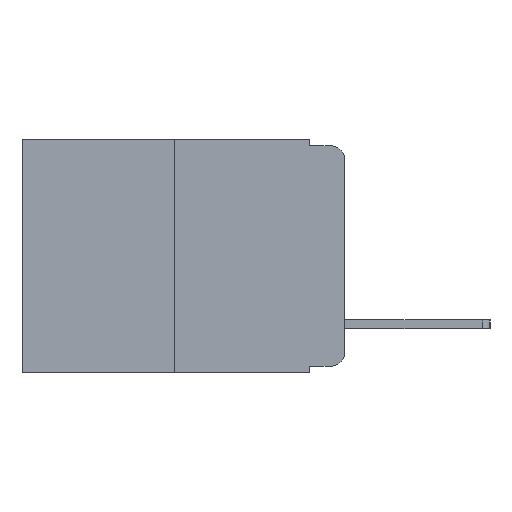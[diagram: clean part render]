
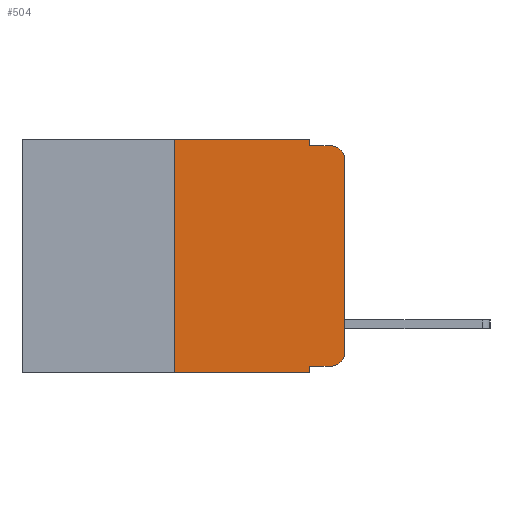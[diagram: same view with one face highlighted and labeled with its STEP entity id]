
A CAD part, left-side view. The second image highlights one B-rep face of the part: STEP entity #504.
In plain terms, the highlighted planar face has unit normal (-1, 0, 0).
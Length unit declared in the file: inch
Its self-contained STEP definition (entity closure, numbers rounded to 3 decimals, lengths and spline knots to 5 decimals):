
#94 = VERTEX_POINT ( 'NONE', #10260 ) ;
#504 = ADVANCED_FACE ( 'NONE', ( #7263 ), #11736, .F. ) ;
#627 = CARTESIAN_POINT ( 'NONE',  ( 0., 0.02, -0.01 ) ) ;
#659 = DIRECTION ( 'NONE',  ( 0., 0., 1. ) ) ;
#711 = CARTESIAN_POINT ( 'NONE',  ( 0., 0.051, 0. ) ) ;
#779 = VERTEX_POINT ( 'NONE', #1316 ) ;
#850 = DIRECTION ( 'NONE',  ( -1., 0., 0. ) ) ;
#1192 = EDGE_CURVE ( 'NONE', #10123, #94, #7740, .T. ) ;
#1227 = CIRCLE ( 'NONE', #11125, 0.02 ) ;
#1251 = VECTOR ( 'NONE', #8469, 39.37008 ) ;
#1261 = CARTESIAN_POINT ( 'NONE',  ( 0., 0., -0.03 ) ) ;
#1316 = CARTESIAN_POINT ( 'NONE',  ( 0., 0.051, -0.343 ) ) ;
#1371 = ORIENTED_EDGE ( 'NONE', *, *, #4126, .F. ) ;
#1494 = DIRECTION ( 'NONE',  ( 0., -1., 0. ) ) ;
#1604 = DIRECTION ( 'NONE',  ( -1., 0., 0. ) ) ;
#1645 = EDGE_LOOP ( 'NONE', ( #10729, #10468, #8356, #1371, #3718, #10208, #5669, #6054, #7855, #7959 ) ) ;
#1779 = VERTEX_POINT ( 'NONE', #7232 ) ;
#2030 = LINE ( 'NONE', #711, #6617 ) ;
#2799 = DIRECTION ( 'NONE',  ( 0., 0., -1. ) ) ;
#2885 = DIRECTION ( 'NONE',  ( 0., 0., -1. ) ) ;
#3276 = VECTOR ( 'NONE', #7156, 39.37008 ) ;
#3371 = EDGE_CURVE ( 'NONE', #8234, #779, #6249, .T. ) ;
#3496 = CARTESIAN_POINT ( 'NONE',  ( 0., 0.473, 0. ) ) ;
#3562 = CARTESIAN_POINT ( 'NONE',  ( 0., 0.051, 0. ) ) ;
#3600 = LINE ( 'NONE', #3562, #3276 ) ;
#3603 = CARTESIAN_POINT ( 'NONE',  ( 0., 0.051, -0.01 ) ) ;
#3718 = ORIENTED_EDGE ( 'NONE', *, *, #1192, .F. ) ;
#4036 = LINE ( 'NONE', #9916, #4349 ) ;
#4106 = EDGE_CURVE ( 'NONE', #11775, #6430, #8516, .T. ) ;
#4109 = EDGE_CURVE ( 'NONE', #6430, #7948, #1227, .T. ) ;
#4125 = EDGE_CURVE ( 'NONE', #11180, #7948, #5952, .T. ) ;
#4126 = EDGE_CURVE ( 'NONE', #94, #11180, #3600, .T. ) ;
#4181 = EDGE_CURVE ( 'NONE', #8234, #10123, #7412, .T. ) ;
#4215 = EDGE_CURVE ( 'NONE', #1779, #779, #2030, .T. ) ;
#4258 = EDGE_CURVE ( 'NONE', #1779, #9437, #4036, .T. ) ;
#4261 = DIRECTION ( 'NONE',  ( 1., 0., 0. ) ) ;
#4275 = EDGE_CURVE ( 'NONE', #9437, #11775, #5815, .T. ) ;
#4349 = VECTOR ( 'NONE', #7314, 39.37008 ) ;
#4845 = CARTESIAN_POINT ( 'NONE',  ( 0., 0.051, -0.01 ) ) ;
#5669 = ORIENTED_EDGE ( 'NONE', *, *, #3371, .T. ) ;
#5742 = VECTOR ( 'NONE', #1494, 39.37008 ) ;
#5815 = CIRCLE ( 'NONE', #8435, 0.02 ) ;
#5952 = LINE ( 'NONE', #3603, #7977 ) ;
#6054 = ORIENTED_EDGE ( 'NONE', *, *, #4215, .F. ) ;
#6249 = LINE ( 'NONE', #7578, #1251 ) ;
#6279 = CARTESIAN_POINT ( 'NONE',  ( 0., 0.25, 0. ) ) ;
#6430 = VERTEX_POINT ( 'NONE', #1261 ) ;
#6514 = CARTESIAN_POINT ( 'NONE',  ( 0., 0.02, -0.313 ) ) ;
#6523 = CARTESIAN_POINT ( 'NONE',  ( 0., 0., -0.313 ) ) ;
#6617 = VECTOR ( 'NONE', #2799, 39.37008 ) ;
#7120 = CARTESIAN_POINT ( 'NONE',  ( 0., 0.02, -0.03 ) ) ;
#7156 = DIRECTION ( 'NONE',  ( 0., 0., -1. ) ) ;
#7232 = CARTESIAN_POINT ( 'NONE',  ( 0., 0.051, -0.333 ) ) ;
#7263 = FACE_OUTER_BOUND ( 'NONE', #1645, .T. ) ;
#7314 = DIRECTION ( 'NONE',  ( 0., -1., 0. ) ) ;
#7381 = DIRECTION ( 'NONE',  ( 0., 0., -1. ) ) ;
#7412 = LINE ( 'NONE', #11472, #11660 ) ;
#7578 = CARTESIAN_POINT ( 'NONE',  ( 0., 0.473, -0.343 ) ) ;
#7740 = LINE ( 'NONE', #3496, #5742 ) ;
#7855 = ORIENTED_EDGE ( 'NONE', *, *, #4258, .T. ) ;
#7948 = VERTEX_POINT ( 'NONE', #627 ) ;
#7955 = DIRECTION ( 'NONE',  ( 0., 0., -1. ) ) ;
#7959 = ORIENTED_EDGE ( 'NONE', *, *, #4275, .T. ) ;
#7977 = VECTOR ( 'NONE', #11377, 39.37008 ) ;
#8234 = VERTEX_POINT ( 'NONE', #10961 ) ;
#8356 = ORIENTED_EDGE ( 'NONE', *, *, #4125, .F. ) ;
#8435 = AXIS2_PLACEMENT_3D ( 'NONE', #6514, #850, #7381 ) ;
#8469 = DIRECTION ( 'NONE',  ( 0., -1., 0. ) ) ;
#8516 = LINE ( 'NONE', #10444, #10491 ) ;
#9193 = AXIS2_PLACEMENT_3D ( 'NONE', #9726, #4261, #2885 ) ;
#9437 = VERTEX_POINT ( 'NONE', #9749 ) ;
#9663 = DIRECTION ( 'NONE',  ( 0., 0., 1. ) ) ;
#9726 = CARTESIAN_POINT ( 'NONE',  ( 0., 0.473, 0. ) ) ;
#9749 = CARTESIAN_POINT ( 'NONE',  ( 0., 0.02, -0.333 ) ) ;
#9916 = CARTESIAN_POINT ( 'NONE',  ( 0., 0.051, -0.333 ) ) ;
#10123 = VERTEX_POINT ( 'NONE', #6279 ) ;
#10208 = ORIENTED_EDGE ( 'NONE', *, *, #4181, .F. ) ;
#10260 = CARTESIAN_POINT ( 'NONE',  ( 0., 0.051, 0. ) ) ;
#10444 = CARTESIAN_POINT ( 'NONE',  ( 0., 0., 0. ) ) ;
#10468 = ORIENTED_EDGE ( 'NONE', *, *, #4109, .T. ) ;
#10491 = VECTOR ( 'NONE', #9663, 39.37008 ) ;
#10729 = ORIENTED_EDGE ( 'NONE', *, *, #4106, .T. ) ;
#10961 = CARTESIAN_POINT ( 'NONE',  ( 0., 0.25, -0.343 ) ) ;
#11125 = AXIS2_PLACEMENT_3D ( 'NONE', #7120, #1604, #7955 ) ;
#11180 = VERTEX_POINT ( 'NONE', #4845 ) ;
#11377 = DIRECTION ( 'NONE',  ( 0., -1., 0. ) ) ;
#11472 = CARTESIAN_POINT ( 'NONE',  ( 0., 0.25, 0. ) ) ;
#11660 = VECTOR ( 'NONE', #659, 39.37008 ) ;
#11736 = PLANE ( 'NONE',  #9193 ) ;
#11775 = VERTEX_POINT ( 'NONE', #6523 ) ;
